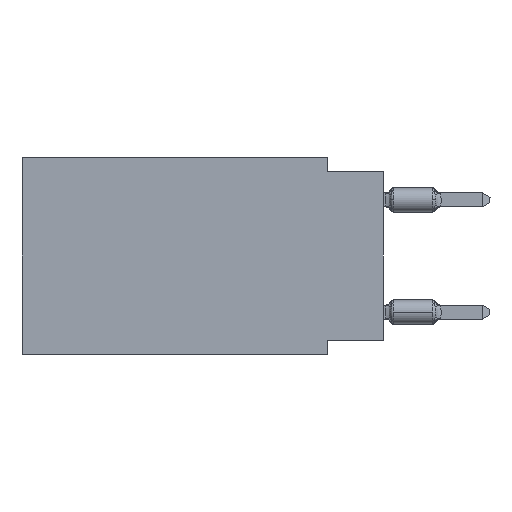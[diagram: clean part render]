
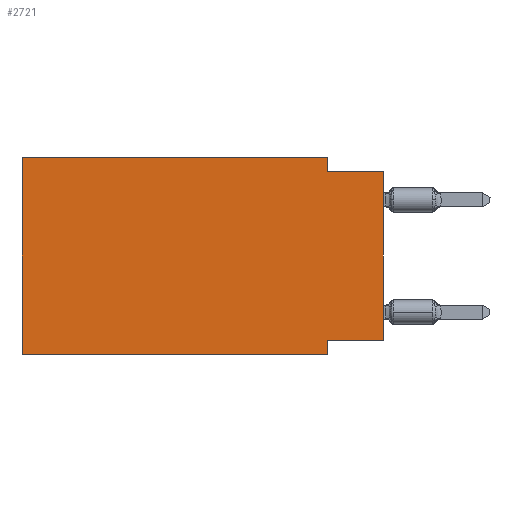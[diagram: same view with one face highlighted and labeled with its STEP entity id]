
A CAD part, left-side view. The second image highlights one B-rep face of the part: STEP entity #2721.
In plain terms, the highlighted planar face has unit normal (-1, 0, 0).
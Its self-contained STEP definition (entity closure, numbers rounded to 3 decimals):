
#304 = ORIENTED_EDGE ( 'NONE', *, *, #24651, .T. ) ;
#708 = ORIENTED_EDGE ( 'NONE', *, *, #14737, .F. ) ;
#964 = DIRECTION ( 'NONE',  ( 0., -1., 0. ) ) ;
#2721 = ADVANCED_FACE ( 'NONE', ( #13011 ), #7411, .F. ) ;
#2852 = VERTEX_POINT ( 'NONE', #13600 ) ;
#3293 = EDGE_CURVE ( 'NONE', #3786, #9169, #22790, .T. ) ;
#3760 = CARTESIAN_POINT ( 'NONE',  ( 0., 16.383, 0. ) ) ;
#3786 = VERTEX_POINT ( 'NONE', #27797 ) ;
#4119 = ORIENTED_EDGE ( 'NONE', *, *, #16653, .F. ) ;
#4425 = CARTESIAN_POINT ( 'NONE',  ( 0., 0., -0.635 ) ) ;
#4710 = ORIENTED_EDGE ( 'NONE', *, *, #10325, .F. ) ;
#6676 = CARTESIAN_POINT ( 'NONE',  ( 0., 2.54, -8.89 ) ) ;
#7007 = VECTOR ( 'NONE', #22079, 1000. ) ;
#7216 = ORIENTED_EDGE ( 'NONE', *, *, #28515, .F. ) ;
#7293 = VECTOR ( 'NONE', #20271, 1000. ) ;
#7374 = CARTESIAN_POINT ( 'NONE',  ( 0., 16.383, 0. ) ) ;
#7411 = PLANE ( 'NONE',  #14048 ) ;
#8790 = CARTESIAN_POINT ( 'NONE',  ( 0., 16.383, -8.89 ) ) ;
#8969 = VECTOR ( 'NONE', #36890, 1000. ) ;
#9169 = VERTEX_POINT ( 'NONE', #19091 ) ;
#10112 = DIRECTION ( 'NONE',  ( 0., 0., -1. ) ) ;
#10325 = EDGE_CURVE ( 'NONE', #2852, #10916, #32611, .T. ) ;
#10916 = VERTEX_POINT ( 'NONE', #36056 ) ;
#11883 = VECTOR ( 'NONE', #28826, 1000. ) ;
#12217 = ORIENTED_EDGE ( 'NONE', *, *, #19513, .F. ) ;
#12841 = VECTOR ( 'NONE', #34326, 1000. ) ;
#13011 = FACE_OUTER_BOUND ( 'NONE', #14237, .T. ) ;
#13078 = CARTESIAN_POINT ( 'NONE',  ( 0., 16.383, 0. ) ) ;
#13600 = CARTESIAN_POINT ( 'NONE',  ( 0., 2.54, 0. ) ) ;
#14048 = AXIS2_PLACEMENT_3D ( 'NONE', #3760, #19216, #10112 ) ;
#14237 = EDGE_LOOP ( 'NONE', ( #21829, #7216, #4710, #4119, #12217, #304, #708, #27532 ) ) ;
#14636 = DIRECTION ( 'NONE',  ( 0., 0., -1. ) ) ;
#14737 = EDGE_CURVE ( 'NONE', #9169, #21945, #16338, .T. ) ;
#14824 = CARTESIAN_POINT ( 'NONE',  ( 0., 2.54, 0. ) ) ;
#16041 = CARTESIAN_POINT ( 'NONE',  ( 0., 16.383, 0. ) ) ;
#16338 = LINE ( 'NONE', #33931, #12841 ) ;
#16653 = EDGE_CURVE ( 'NONE', #18727, #2852, #33977, .T. ) ;
#17834 = VECTOR ( 'NONE', #14636, 1000. ) ;
#18727 = VERTEX_POINT ( 'NONE', #16041 ) ;
#19091 = CARTESIAN_POINT ( 'NONE',  ( 0., 2.54, -8.255 ) ) ;
#19216 = DIRECTION ( 'NONE',  ( 1., 0., 0. ) ) ;
#19513 = EDGE_CURVE ( 'NONE', #24699, #18727, #30763, .T. ) ;
#20271 = DIRECTION ( 'NONE',  ( 0., 1., 0. ) ) ;
#21829 = ORIENTED_EDGE ( 'NONE', *, *, #26625, .T. ) ;
#21945 = VERTEX_POINT ( 'NONE', #6676 ) ;
#22079 = DIRECTION ( 'NONE',  ( 0., 0., 1. ) ) ;
#22790 = LINE ( 'NONE', #35356, #7293 ) ;
#22932 = LINE ( 'NONE', #34729, #26062 ) ;
#24263 = DIRECTION ( 'NONE',  ( 0., -1., 0. ) ) ;
#24651 = EDGE_CURVE ( 'NONE', #24699, #21945, #22932, .T. ) ;
#24699 = VERTEX_POINT ( 'NONE', #8790 ) ;
#25796 = VERTEX_POINT ( 'NONE', #26226 ) ;
#26062 = VECTOR ( 'NONE', #24263, 1000. ) ;
#26132 = CARTESIAN_POINT ( 'NONE',  ( 0., 0., 0. ) ) ;
#26226 = CARTESIAN_POINT ( 'NONE',  ( 0., 0., -0.635 ) ) ;
#26625 = EDGE_CURVE ( 'NONE', #3786, #25796, #35034, .T. ) ;
#27532 = ORIENTED_EDGE ( 'NONE', *, *, #3293, .F. ) ;
#27797 = CARTESIAN_POINT ( 'NONE',  ( 0., 0., -8.255 ) ) ;
#28515 = EDGE_CURVE ( 'NONE', #10916, #25796, #30706, .T. ) ;
#28826 = DIRECTION ( 'NONE',  ( 0., 0., 1. ) ) ;
#30706 = LINE ( 'NONE', #4425, #33580 ) ;
#30763 = LINE ( 'NONE', #7374, #7007 ) ;
#32611 = LINE ( 'NONE', #14824, #17834 ) ;
#33580 = VECTOR ( 'NONE', #964, 1000. ) ;
#33931 = CARTESIAN_POINT ( 'NONE',  ( 0., 2.54, -8.89 ) ) ;
#33977 = LINE ( 'NONE', #13078, #8969 ) ;
#34326 = DIRECTION ( 'NONE',  ( 0., 0., -1. ) ) ;
#34729 = CARTESIAN_POINT ( 'NONE',  ( 0., 16.383, -8.89 ) ) ;
#35034 = LINE ( 'NONE', #26132, #11883 ) ;
#35356 = CARTESIAN_POINT ( 'NONE',  ( 0., 0., -8.255 ) ) ;
#36056 = CARTESIAN_POINT ( 'NONE',  ( 0., 2.54, -0.635 ) ) ;
#36890 = DIRECTION ( 'NONE',  ( 0., -1., 0. ) ) ;
